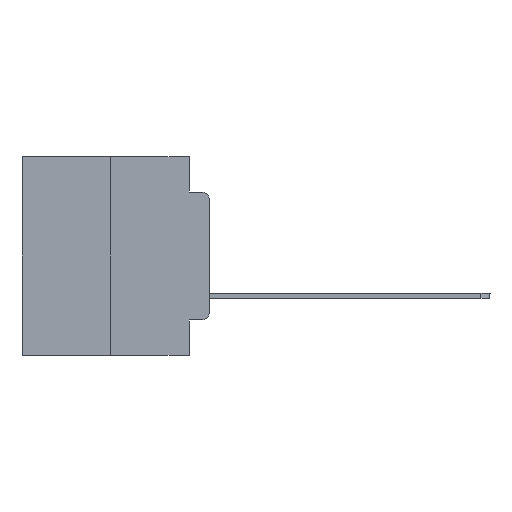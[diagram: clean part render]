
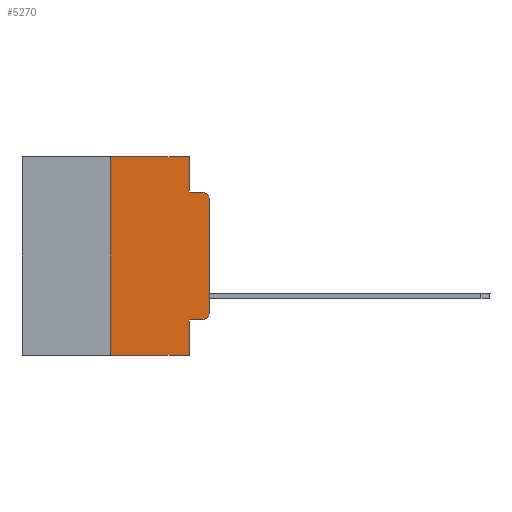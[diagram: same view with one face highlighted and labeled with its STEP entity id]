
A CAD part, left-side view. The second image highlights one B-rep face of the part: STEP entity #5270.
In plain terms, the highlighted planar face has unit normal (-1, 0, 0).
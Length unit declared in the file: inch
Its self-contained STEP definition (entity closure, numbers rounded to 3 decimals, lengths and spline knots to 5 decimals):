
#397 = CIRCLE ( 'NONE', #15795, 0.02 ) ;
#858 = CARTESIAN_POINT ( 'NONE',  ( 0., 0.02, -0.4115 ) ) ;
#1021 = VECTOR ( 'NONE', #11273, 39.37008 ) ;
#1089 = CARTESIAN_POINT ( 'NONE',  ( 0., 0.051, -0.4115 ) ) ;
#1378 = DIRECTION ( 'NONE',  ( 0., -1., 0. ) ) ;
#2110 = LINE ( 'NONE', #26586, #2111 ) ;
#2111 = VECTOR ( 'NONE', #24519, 39.37008 ) ;
#2218 = EDGE_CURVE ( 'NONE', #19713, #20926, #2110, .T. ) ;
#2444 = VERTEX_POINT ( 'NONE', #858 ) ;
#3242 = ORIENTED_EDGE ( 'NONE', *, *, #6869, .F. ) ;
#3815 = DIRECTION ( 'NONE',  ( 0., 0., -1. ) ) ;
#4218 = CARTESIAN_POINT ( 'NONE',  ( 0., 0.02, -0.1085 ) ) ;
#4403 = ORIENTED_EDGE ( 'NONE', *, *, #22773, .T. ) ;
#4893 = VECTOR ( 'NONE', #1378, 39.37008 ) ;
#5270 = ADVANCED_FACE ( 'NONE', ( #10540 ), #10686, .F. ) ;
#5934 = DIRECTION ( 'NONE',  ( 0., -1., 0. ) ) ;
#6694 = VECTOR ( 'NONE', #23623, 39.37008 ) ;
#6838 = EDGE_CURVE ( 'NONE', #7189, #8196, #14170, .T. ) ;
#6869 = EDGE_CURVE ( 'NONE', #20926, #7189, #22532, .T. ) ;
#7189 = VERTEX_POINT ( 'NONE', #17566 ) ;
#8196 = VERTEX_POINT ( 'NONE', #24474 ) ;
#8364 = VERTEX_POINT ( 'NONE', #20756 ) ;
#8383 = CARTESIAN_POINT ( 'NONE',  ( 0., 0.25, 0. ) ) ;
#9119 = CARTESIAN_POINT ( 'NONE',  ( 0., 0.051, -0.4115 ) ) ;
#9693 = VERTEX_POINT ( 'NONE', #1089 ) ;
#9781 = ORIENTED_EDGE ( 'NONE', *, *, #17964, .T. ) ;
#9913 = CARTESIAN_POINT ( 'NONE',  ( 0., 0.473, 0. ) ) ;
#9916 = CARTESIAN_POINT ( 'NONE',  ( 0., 0.473, -0.5 ) ) ;
#10540 = FACE_OUTER_BOUND ( 'NONE', #16674, .T. ) ;
#10686 = PLANE ( 'NONE',  #23857 ) ;
#11137 = LINE ( 'NONE', #23905, #1021 ) ;
#11258 = CARTESIAN_POINT ( 'NONE',  ( 0., 0.25, -0.5 ) ) ;
#11273 = DIRECTION ( 'NONE',  ( 0., 0., -1. ) ) ;
#11320 = EDGE_CURVE ( 'NONE', #19713, #11710, #22400, .T. ) ;
#11413 = CIRCLE ( 'NONE', #26314, 0.02 ) ;
#11600 = EDGE_CURVE ( 'NONE', #9693, #11710, #11137, .T. ) ;
#11678 = ORIENTED_EDGE ( 'NONE', *, *, #21379, .T. ) ;
#11710 = VERTEX_POINT ( 'NONE', #16477 ) ;
#12003 = VERTEX_POINT ( 'NONE', #21673 ) ;
#12108 = DIRECTION ( 'NONE',  ( 0., 0., -1. ) ) ;
#12253 = ORIENTED_EDGE ( 'NONE', *, *, #2218, .F. ) ;
#13055 = ORIENTED_EDGE ( 'NONE', *, *, #6838, .F. ) ;
#13547 = VERTEX_POINT ( 'NONE', #20826 ) ;
#13744 = ORIENTED_EDGE ( 'NONE', *, *, #25329, .T. ) ;
#14170 = LINE ( 'NONE', #24742, #19793 ) ;
#15080 = VECTOR ( 'NONE', #5934, 39.37008 ) ;
#15094 = DIRECTION ( 'NONE',  ( 1., 0., 0. ) ) ;
#15533 = VECTOR ( 'NONE', #26666, 39.37008 ) ;
#15795 = AXIS2_PLACEMENT_3D ( 'NONE', #4218, #16597, #3815 ) ;
#16465 = ORIENTED_EDGE ( 'NONE', *, *, #11320, .T. ) ;
#16477 = CARTESIAN_POINT ( 'NONE',  ( 0., 0.051, -0.5 ) ) ;
#16597 = DIRECTION ( 'NONE',  ( -1., 0., 0. ) ) ;
#16674 = EDGE_LOOP ( 'NONE', ( #13744, #4403, #23009, #13055, #3242, #12253, #16465, #20742, #9781, #11678 ) ) ;
#16728 = DIRECTION ( 'NONE',  ( 0., 0., -1. ) ) ;
#16869 = DIRECTION ( 'NONE',  ( -1., 0., 0. ) ) ;
#17052 = LINE ( 'NONE', #21007, #6694 ) ;
#17483 = VECTOR ( 'NONE', #17511, 39.37008 ) ;
#17511 = DIRECTION ( 'NONE',  ( 0., -1., 0. ) ) ;
#17566 = CARTESIAN_POINT ( 'NONE',  ( 0., 0.051, 0. ) ) ;
#17964 = EDGE_CURVE ( 'NONE', #9693, #2444, #19962, .T. ) ;
#18301 = LINE ( 'NONE', #24884, #15080 ) ;
#19713 = VERTEX_POINT ( 'NONE', #11258 ) ;
#19793 = VECTOR ( 'NONE', #12108, 39.37008 ) ;
#19962 = LINE ( 'NONE', #9119, #17483 ) ;
#20742 = ORIENTED_EDGE ( 'NONE', *, *, #11600, .F. ) ;
#20756 = CARTESIAN_POINT ( 'NONE',  ( 0., 0., -0.3915 ) ) ;
#20826 = CARTESIAN_POINT ( 'NONE',  ( 0., 0., -0.1085 ) ) ;
#20926 = VERTEX_POINT ( 'NONE', #8383 ) ;
#21007 = CARTESIAN_POINT ( 'NONE',  ( 0., 0., 0. ) ) ;
#21379 = EDGE_CURVE ( 'NONE', #2444, #8364, #11413, .T. ) ;
#21673 = CARTESIAN_POINT ( 'NONE',  ( 0., 0.02, -0.0885 ) ) ;
#22400 = LINE ( 'NONE', #9916, #15533 ) ;
#22532 = LINE ( 'NONE', #9913, #4893 ) ;
#22773 = EDGE_CURVE ( 'NONE', #13547, #12003, #397, .T. ) ;
#23009 = ORIENTED_EDGE ( 'NONE', *, *, #26384, .F. ) ;
#23623 = DIRECTION ( 'NONE',  ( 0., 0., 1. ) ) ;
#23857 = AXIS2_PLACEMENT_3D ( 'NONE', #25110, #15094, #25242 ) ;
#23905 = CARTESIAN_POINT ( 'NONE',  ( 0., 0.051, 0. ) ) ;
#24474 = CARTESIAN_POINT ( 'NONE',  ( 0., 0.051, -0.0885 ) ) ;
#24519 = DIRECTION ( 'NONE',  ( 0., 0., 1. ) ) ;
#24692 = CARTESIAN_POINT ( 'NONE',  ( 0., 0.02, -0.3915 ) ) ;
#24742 = CARTESIAN_POINT ( 'NONE',  ( 0., 0.051, 0. ) ) ;
#24884 = CARTESIAN_POINT ( 'NONE',  ( 0., 0.051, -0.0885 ) ) ;
#25110 = CARTESIAN_POINT ( 'NONE',  ( 0., 0.473, 0. ) ) ;
#25242 = DIRECTION ( 'NONE',  ( 0., 0., -1. ) ) ;
#25329 = EDGE_CURVE ( 'NONE', #8364, #13547, #17052, .T. ) ;
#26314 = AXIS2_PLACEMENT_3D ( 'NONE', #24692, #16869, #16728 ) ;
#26384 = EDGE_CURVE ( 'NONE', #8196, #12003, #18301, .T. ) ;
#26586 = CARTESIAN_POINT ( 'NONE',  ( 0., 0.25, 0. ) ) ;
#26666 = DIRECTION ( 'NONE',  ( 0., -1., 0. ) ) ;
